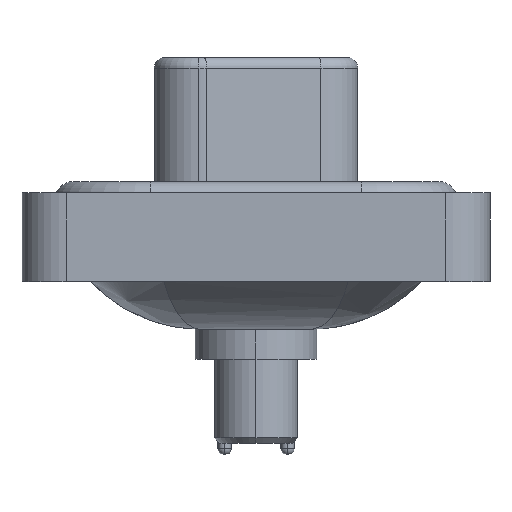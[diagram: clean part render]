
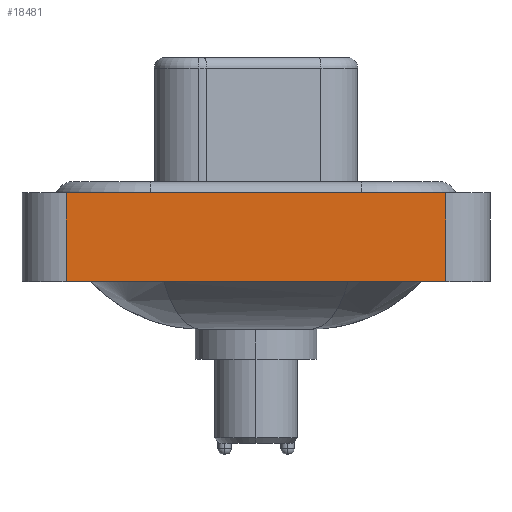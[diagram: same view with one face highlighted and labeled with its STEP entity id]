
A CAD part, left-side view. The second image highlights one B-rep face of the part: STEP entity #18481.
In plain terms, the highlighted planar face has unit normal (-1, 0, 0).
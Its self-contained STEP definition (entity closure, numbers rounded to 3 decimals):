
#174 = DIRECTION ( 'NONE',  ( 0., 0., 1. ) ) ;
#1139 = VERTEX_POINT ( 'NONE', #5285 ) ;
#1404 = CARTESIAN_POINT ( 'NONE',  ( -7.3, -8.55, -3.6 ) ) ;
#1854 = VECTOR ( 'NONE', #12206, 1000. ) ;
#2190 = DIRECTION ( 'NONE',  ( 0., 0., 1. ) ) ;
#3269 = EDGE_CURVE ( 'NONE', #17817, #7815, #12380, .T. ) ;
#3552 = CARTESIAN_POINT ( 'NONE',  ( -7.3, -8.55, -3.6 ) ) ;
#4009 = CARTESIAN_POINT ( 'NONE',  ( -7.3, -8.55, -3.6 ) ) ;
#4214 = LINE ( 'NONE', #1404, #14941 ) ;
#4881 = CARTESIAN_POINT ( 'NONE',  ( -7.3, 8.55, -3.6 ) ) ;
#5048 = EDGE_LOOP ( 'NONE', ( #16540, #8564, #5121, #14843 ) ) ;
#5121 = ORIENTED_EDGE ( 'NONE', *, *, #17753, .F. ) ;
#5285 = CARTESIAN_POINT ( 'NONE',  ( -7.3, 8.55, 0.4 ) ) ;
#6623 = LINE ( 'NONE', #4881, #11772 ) ;
#7815 = VERTEX_POINT ( 'NONE', #14093 ) ;
#8564 = ORIENTED_EDGE ( 'NONE', *, *, #17652, .F. ) ;
#10050 = EDGE_CURVE ( 'NONE', #13304, #17817, #4214, .T. ) ;
#10836 = DIRECTION ( 'NONE',  ( 0., 0., 1. ) ) ;
#10888 = CARTESIAN_POINT ( 'NONE',  ( -7.3, 8.55, -3.6 ) ) ;
#11722 = DIRECTION ( 'NONE',  ( 0., -1., 0. ) ) ;
#11772 = VECTOR ( 'NONE', #10836, 1000. ) ;
#11796 = VECTOR ( 'NONE', #174, 1000. ) ;
#12138 = FACE_OUTER_BOUND ( 'NONE', #5048, .T. ) ;
#12206 = DIRECTION ( 'NONE',  ( 0., -1., 0. ) ) ;
#12380 = LINE ( 'NONE', #16504, #11796 ) ;
#13304 = VERTEX_POINT ( 'NONE', #10888 ) ;
#13742 = LINE ( 'NONE', #15200, #1854 ) ;
#14093 = CARTESIAN_POINT ( 'NONE',  ( -7.3, -8.55, 0.4 ) ) ;
#14843 = ORIENTED_EDGE ( 'NONE', *, *, #10050, .T. ) ;
#14941 = VECTOR ( 'NONE', #11722, 1000. ) ;
#15200 = CARTESIAN_POINT ( 'NONE',  ( -7.3, -8.55, 0.4 ) ) ;
#15514 = DIRECTION ( 'NONE',  ( -1., 0., 0. ) ) ;
#16125 = AXIS2_PLACEMENT_3D ( 'NONE', #3552, #15514, #2190 ) ;
#16504 = CARTESIAN_POINT ( 'NONE',  ( -7.3, -8.55, -3.6 ) ) ;
#16540 = ORIENTED_EDGE ( 'NONE', *, *, #3269, .T. ) ;
#17652 = EDGE_CURVE ( 'NONE', #1139, #7815, #13742, .T. ) ;
#17753 = EDGE_CURVE ( 'NONE', #13304, #1139, #6623, .T. ) ;
#17817 = VERTEX_POINT ( 'NONE', #4009 ) ;
#18057 = PLANE ( 'NONE',  #16125 ) ;
#18481 = ADVANCED_FACE ( 'NONE', ( #12138 ), #18057, .T. ) ;
